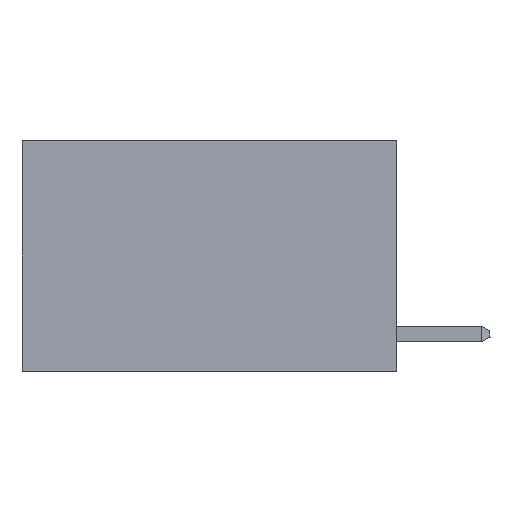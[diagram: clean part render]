
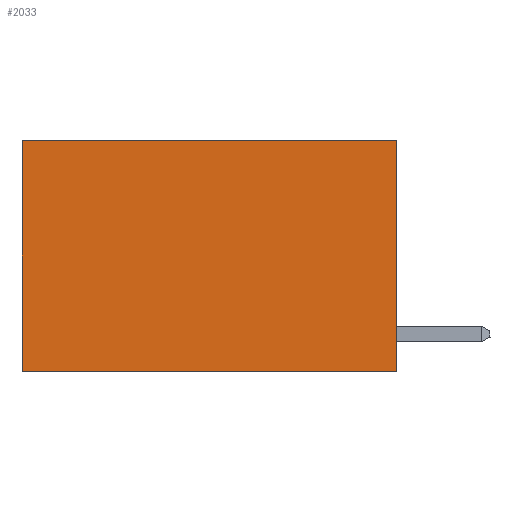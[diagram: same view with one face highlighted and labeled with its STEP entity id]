
A CAD part, left-side view. The second image highlights one B-rep face of the part: STEP entity #2033.
In plain terms, the highlighted planar face has unit normal (-1, 0, 0).
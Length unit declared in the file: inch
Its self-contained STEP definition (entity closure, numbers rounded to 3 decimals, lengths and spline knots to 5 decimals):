
#355 = LINE ( 'NONE', #1471, #14712 ) ;
#743 = EDGE_LOOP ( 'NONE', ( #3513, #11170, #15381, #15827 ) ) ;
#1267 = DIRECTION ( 'NONE',  ( 0., 1., 0. ) ) ;
#1471 = CARTESIAN_POINT ( 'NONE',  ( 0.2625, 0., 0. ) ) ;
#1941 = AXIS2_PLACEMENT_3D ( 'NONE', #16072, #13342, #12982 ) ;
#1952 = VECTOR ( 'NONE', #1267, 39.37008 ) ;
#2033 = ADVANCED_FACE ( 'NONE', ( #8153 ), #14437, .F. ) ;
#3169 = DIRECTION ( 'NONE',  ( 0., 0., -1. ) ) ;
#3513 = ORIENTED_EDGE ( 'NONE', *, *, #5160, .T. ) ;
#4028 = LINE ( 'NONE', #6110, #11241 ) ;
#4109 = CARTESIAN_POINT ( 'NONE',  ( 0.2625, 0., -0.37 ) ) ;
#4362 = DIRECTION ( 'NONE',  ( 0., 0., -1. ) ) ;
#4980 = EDGE_CURVE ( 'NONE', #11641, #6231, #9600, .T. ) ;
#5160 = EDGE_CURVE ( 'NONE', #14508, #6231, #17791, .T. ) ;
#6003 = CARTESIAN_POINT ( 'NONE',  ( 0.2625, 0.6, 0. ) ) ;
#6110 = CARTESIAN_POINT ( 'NONE',  ( 0.2625, 0., 0. ) ) ;
#6231 = VERTEX_POINT ( 'NONE', #12769 ) ;
#8153 = FACE_OUTER_BOUND ( 'NONE', #743, .T. ) ;
#9216 = EDGE_CURVE ( 'NONE', #17650, #11641, #355, .T. ) ;
#9600 = LINE ( 'NONE', #4109, #1952 ) ;
#11170 = ORIENTED_EDGE ( 'NONE', *, *, #4980, .F. ) ;
#11241 = VECTOR ( 'NONE', #14730, 39.37008 ) ;
#11641 = VERTEX_POINT ( 'NONE', #13182 ) ;
#12769 = CARTESIAN_POINT ( 'NONE',  ( 0.2625, 0.6, -0.37 ) ) ;
#12982 = DIRECTION ( 'NONE',  ( 0., 0., -1. ) ) ;
#13182 = CARTESIAN_POINT ( 'NONE',  ( 0.2625, 0., -0.37 ) ) ;
#13342 = DIRECTION ( 'NONE',  ( 1., 0., 0. ) ) ;
#13573 = VECTOR ( 'NONE', #3169, 39.37008 ) ;
#14177 = EDGE_CURVE ( 'NONE', #17650, #14508, #4028, .T. ) ;
#14437 = PLANE ( 'NONE',  #1941 ) ;
#14508 = VERTEX_POINT ( 'NONE', #16820 ) ;
#14712 = VECTOR ( 'NONE', #4362, 39.37008 ) ;
#14730 = DIRECTION ( 'NONE',  ( 0., 1., 0. ) ) ;
#15381 = ORIENTED_EDGE ( 'NONE', *, *, #9216, .F. ) ;
#15824 = CARTESIAN_POINT ( 'NONE',  ( 0.2625, 0., 0. ) ) ;
#15827 = ORIENTED_EDGE ( 'NONE', *, *, #14177, .T. ) ;
#16072 = CARTESIAN_POINT ( 'NONE',  ( 0.2625, 0., 0. ) ) ;
#16820 = CARTESIAN_POINT ( 'NONE',  ( 0.2625, 0.6, 0. ) ) ;
#17650 = VERTEX_POINT ( 'NONE', #15824 ) ;
#17791 = LINE ( 'NONE', #6003, #13573 ) ;
